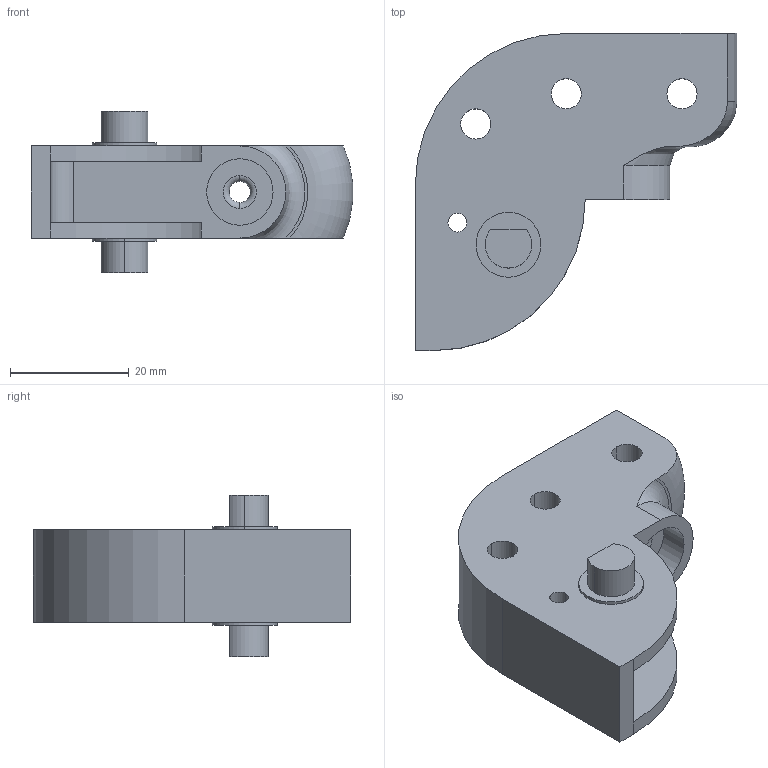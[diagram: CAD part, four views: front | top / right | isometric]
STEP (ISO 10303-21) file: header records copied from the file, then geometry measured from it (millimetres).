
FILE_DESCRIPTION (( 'STEP AP214' ), '1' );
FILE_NAME ('hammer body.STEP', '2013-05-27T22:43:30', ( 'Asher' ), ( '' ), 'SwSTEP 2.0', 'SolidWorks 2013', '' );
FILE_SCHEMA (( 'AUTOMOTIVE_DESIGN' ));
Length unit declared in the file: millimetre
Products named in the file (1): hammer body
Bounding box: 54.06 x 53.34 x 27.18 mm (x, y, z)
Volume: 21906 mm3; surface area: 8919.2 mm2
Topology: 1 solids, 1 shells, 50 faces, 125 edges, 82 vertices
Faces by surface type: cylinder 29, plane 17, torus 4
Entity records: 1637 total; most frequent: CARTESIAN_POINT 324, DIRECTION 287, ORIENTED_EDGE 250, EDGE_CURVE 125, AXIS2_PLACEMENT_3D 115, VERTEX_POINT 82, EDGE_LOOP 67, CIRCLE 64
